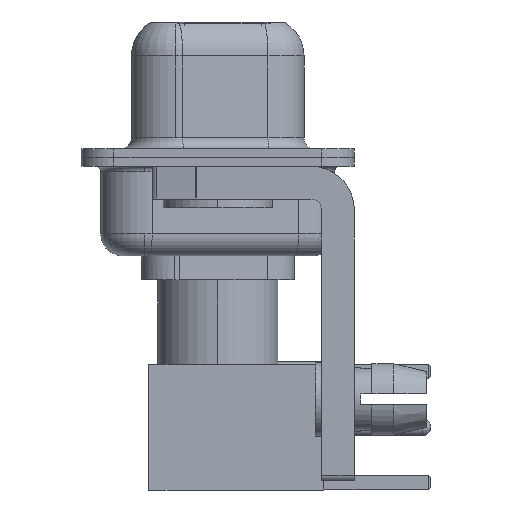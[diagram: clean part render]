
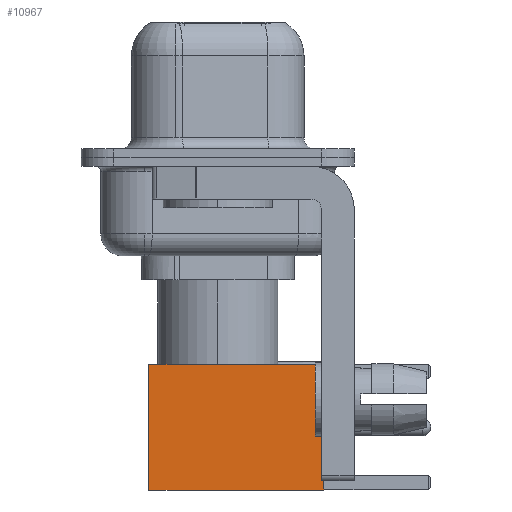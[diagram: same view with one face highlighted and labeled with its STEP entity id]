
A CAD part, left-side view. The second image highlights one B-rep face of the part: STEP entity #10967.
In plain terms, the highlighted face is planar.
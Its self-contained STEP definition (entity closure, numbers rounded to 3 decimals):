
#770 = VERTEX_POINT ( 'NONE', #14234 ) ;
#1700 = CARTESIAN_POINT ( 'NONE',  ( 2.875, 2.875, 0. ) ) ;
#2549 = DIRECTION ( 'NONE',  ( 0., 0., 1. ) ) ;
#3130 = CARTESIAN_POINT ( 'NONE',  ( -2.875, 2.875, 8. ) ) ;
#3552 = DIRECTION ( 'NONE',  ( -1., 0., 0. ) ) ;
#3899 = CARTESIAN_POINT ( 'NONE',  ( 0., 2.875, 8. ) ) ;
#4498 = EDGE_CURVE ( 'NONE', #770, #5989, #17424, .T. ) ;
#5246 = CARTESIAN_POINT ( 'NONE',  ( -2.875, 2.875, 0. ) ) ;
#5989 = VERTEX_POINT ( 'NONE', #5246 ) ;
#6573 = ORIENTED_EDGE ( 'NONE', *, *, #12359, .F. ) ;
#7845 = PLANE ( 'NONE',  #13631 ) ;
#7955 = CARTESIAN_POINT ( 'NONE',  ( 2.875, 2.875, 0. ) ) ;
#8298 = VERTEX_POINT ( 'NONE', #3130 ) ;
#8466 = LINE ( 'NONE', #1700, #8810 ) ;
#8699 = CARTESIAN_POINT ( 'NONE',  ( 0., 2.875, 0. ) ) ;
#8810 = VECTOR ( 'NONE', #10077, 1000. ) ;
#8891 = CARTESIAN_POINT ( 'NONE',  ( -2.875, 2.875, 0. ) ) ;
#9233 = LINE ( 'NONE', #8891, #11857 ) ;
#10077 = DIRECTION ( 'NONE',  ( 0., 0., -1. ) ) ;
#10493 = VECTOR ( 'NONE', #3552, 1000. ) ;
#10967 = ADVANCED_FACE ( 'NONE', ( #14842 ), #7845, .T. ) ;
#11267 = DIRECTION ( 'NONE',  ( 0., 1., 0. ) ) ;
#11857 = VECTOR ( 'NONE', #14390, 1000. ) ;
#12359 = EDGE_CURVE ( 'NONE', #8298, #5989, #9233, .T. ) ;
#13631 = AXIS2_PLACEMENT_3D ( 'NONE', #7955, #11267, #2549 ) ;
#14234 = CARTESIAN_POINT ( 'NONE',  ( 2.875, 2.875, 0. ) ) ;
#14390 = DIRECTION ( 'NONE',  ( 0., 0., -1. ) ) ;
#14810 = EDGE_CURVE ( 'NONE', #22359, #8298, #19314, .T. ) ;
#14842 = FACE_OUTER_BOUND ( 'NONE', #21723, .T. ) ;
#14866 = ORIENTED_EDGE ( 'NONE', *, *, #14810, .F. ) ;
#15001 = VECTOR ( 'NONE', #17658, 1000. ) ;
#15551 = CARTESIAN_POINT ( 'NONE',  ( 2.875, 2.875, 8. ) ) ;
#17424 = LINE ( 'NONE', #8699, #15001 ) ;
#17658 = DIRECTION ( 'NONE',  ( -1., 0., 0. ) ) ;
#18109 = EDGE_CURVE ( 'NONE', #22359, #770, #8466, .T. ) ;
#19314 = LINE ( 'NONE', #3899, #10493 ) ;
#20707 = ORIENTED_EDGE ( 'NONE', *, *, #4498, .T. ) ;
#21723 = EDGE_LOOP ( 'NONE', ( #22415, #20707, #6573, #14866 ) ) ;
#22359 = VERTEX_POINT ( 'NONE', #15551 ) ;
#22415 = ORIENTED_EDGE ( 'NONE', *, *, #18109, .T. ) ;
